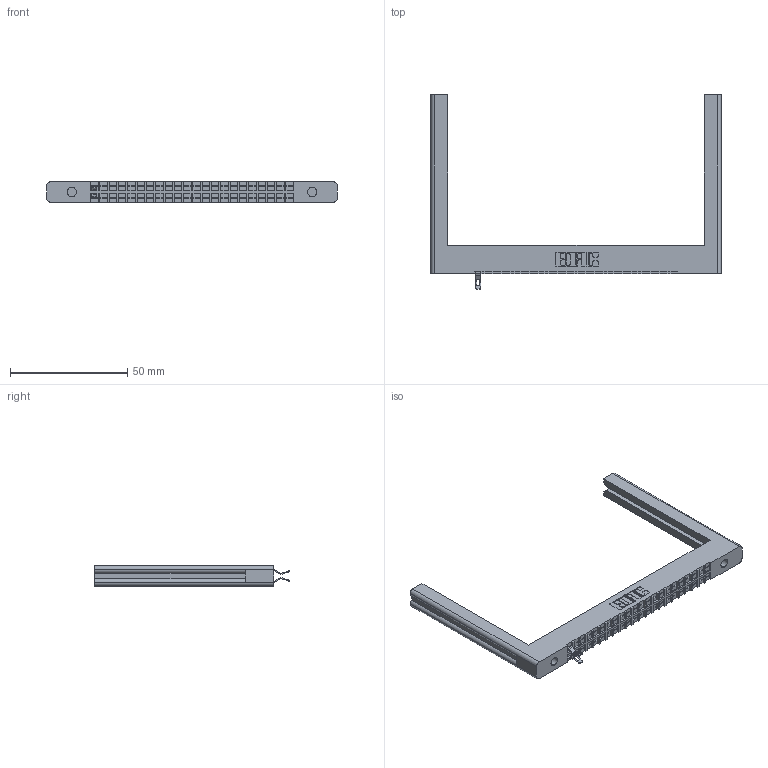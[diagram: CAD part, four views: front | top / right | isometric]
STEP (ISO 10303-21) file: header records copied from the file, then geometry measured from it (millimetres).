
FILE_DESCRIPTION (( 'STEP AP203' ), '1' );
FILE_NAME ('322-044-555-254.STEP', '2018-08-01T11:38:27', ( '' ), ( '' ), 'SwSTEP 2.0', 'SolidWorks 2016', '' );
FILE_SCHEMA (( 'CONFIG_CONTROL_DESIGN' ));
Length unit declared in the file: inch
Products named in the file (3): 322-044-555-254; 322 Part; 307-290-001_555
Assembly tree (3 placements, depth 2):
  322-044-555-254
    322 Part
    307-290-001_555  x2
Bounding box: 123.83 x 82.93 x 8.71 mm (x, y, z)
Volume: 15525.7 mm3; surface area: 14345.5 mm2
Topology: 3 solids, 3 shells, 687 faces, 2151 edges, 1430 vertices
Faces by surface type: plane 543, cylinder 144
Entity records: 22467 total; most frequent: ORIENTED_EDGE 4004, CARTESIAN_POINT 3976, DIRECTION 3528, EDGE_CURVE 2002, LINE 1760, VECTOR 1760, VERTEX_POINT 1332, AXIS2_PLACEMENT_3D 884
